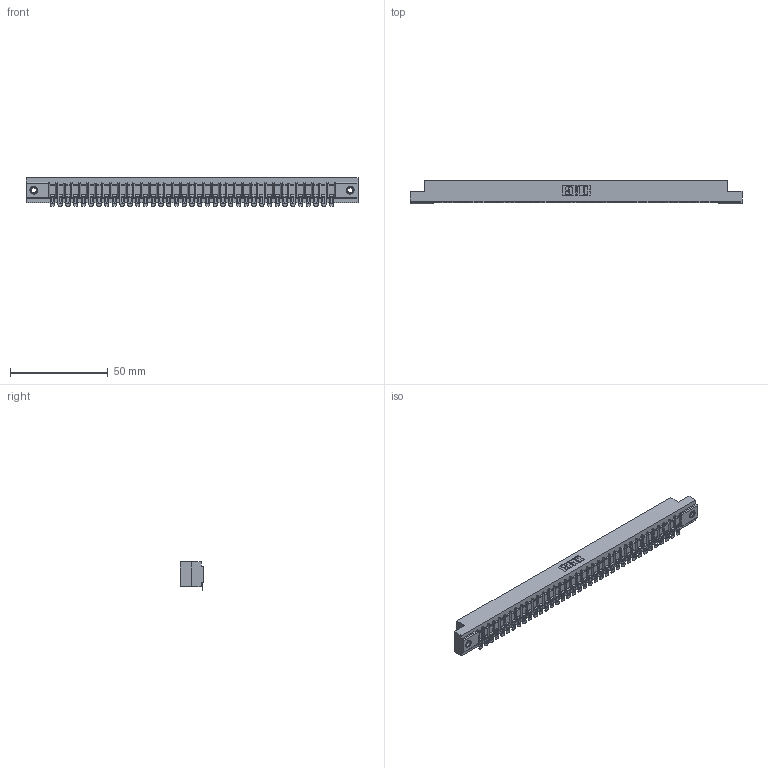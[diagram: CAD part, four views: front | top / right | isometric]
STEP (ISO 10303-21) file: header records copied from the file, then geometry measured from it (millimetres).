
FILE_DESCRIPTION (( 'STEP AP203' ), '1' );
FILE_NAME ('307-037-554-107.STEP', '2019-09-05T08:39:44', ( '' ), ( '' ), 'SwSTEP 2.0', 'SolidWorks 2016', '' );
FILE_SCHEMA (( 'CONFIG_CONTROL_DESIGN' ));
Length unit declared in the file: inch
Products named in the file (4): 307 Part_.156 Dia Mounting Holes; 345-250-001_345-250-005-103; 307-037-554-107; 307-290-002_554
Assembly tree (40 placements, depth 2):
  307-037-554-107
    307 Part_.156 Dia Mounting Holes
    307-290-002_554  x37
    345-250-001_345-250-005-103  x2
Bounding box: 169.62 x 12.01 x 14.52 mm (x, y, z)
Volume: 18114.1 mm3; surface area: 22841.5 mm2
Topology: 40 solids, 40 shells, 3213 faces, 9820 edges, 6436 vertices
Faces by surface type: plane 1804, cylinder 1317, sphere 76, cone 12, torus 4
Entity records: 34486 total; most frequent: CARTESIAN_POINT 5797, ORIENTED_EDGE 5780, DIRECTION 5650, EDGE_CURVE 2890, VECTOR 2204, LINE 2204, VERTEX_POINT 1870, AXIS2_PLACEMENT_3D 1723
